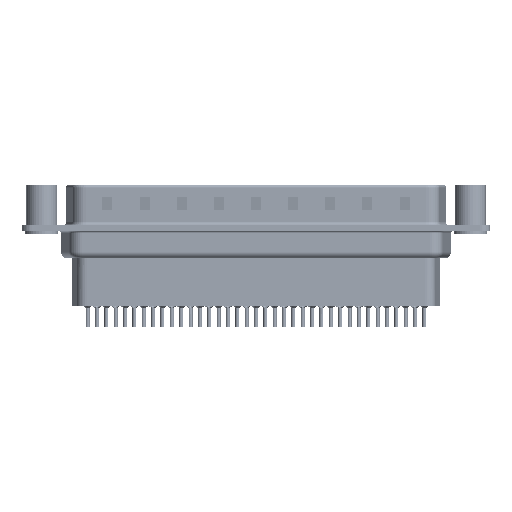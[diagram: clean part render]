
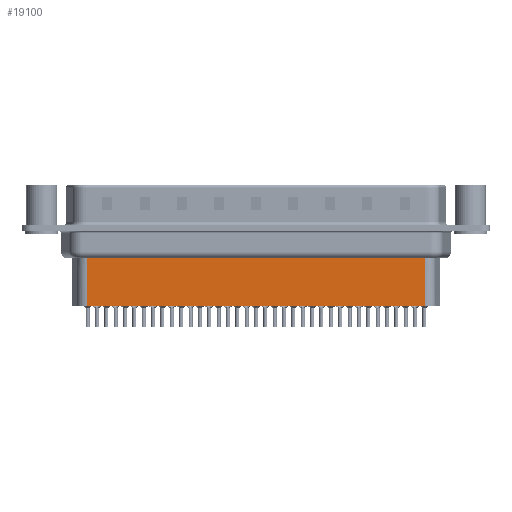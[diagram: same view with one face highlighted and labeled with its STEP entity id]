
A CAD part, front view. The second image highlights one B-rep face of the part: STEP entity #19100.
In plain terms, the highlighted planar face has unit normal (0, -1, 0).
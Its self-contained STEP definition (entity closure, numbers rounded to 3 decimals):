
#1146 = EDGE_LOOP ( 'NONE', ( #26297, #23193, #11882, #1298 ) ) ;
#1298 = ORIENTED_EDGE ( 'NONE', *, *, #6288, .F. ) ;
#3890 = VECTOR ( 'NONE', #13657, 1000. ) ;
#3902 = CARTESIAN_POINT ( 'NONE',  ( 6.706, -3.5, -3.1 ) ) ;
#4260 = CARTESIAN_POINT ( 'NONE',  ( 6.706, -3.5, -4.097 ) ) ;
#4606 = LINE ( 'NONE', #11384, #3890 ) ;
#4871 = CARTESIAN_POINT ( 'NONE',  ( 6.706, -3.5, -11.45 ) ) ;
#5815 = VERTEX_POINT ( 'NONE', #4260 ) ;
#6288 = EDGE_CURVE ( 'NONE', #29501, #21050, #11041, .T. ) ;
#6934 = CARTESIAN_POINT ( 'NONE',  ( 6.706, -3.5, -11.45 ) ) ;
#8569 = DIRECTION ( 'NONE',  ( 0., -1., 0. ) ) ;
#11041 = LINE ( 'NONE', #4871, #16388 ) ;
#11384 = CARTESIAN_POINT ( 'NONE',  ( 6.706, -3.5, -3.1 ) ) ;
#11430 = DIRECTION ( 'NONE',  ( 0., 0., -1. ) ) ;
#11882 = ORIENTED_EDGE ( 'NONE', *, *, #25477, .T. ) ;
#12043 = LINE ( 'NONE', #16840, #17436 ) ;
#12230 = DIRECTION ( 'NONE',  ( -1., 0., 0. ) ) ;
#13657 = DIRECTION ( 'NONE',  ( 0., 0., -1. ) ) ;
#13938 = LINE ( 'NONE', #25415, #26463 ) ;
#16388 = VECTOR ( 'NONE', #23358, 1000. ) ;
#16840 = CARTESIAN_POINT ( 'NONE',  ( 6.459, -3.5, -4.097 ) ) ;
#17436 = VECTOR ( 'NONE', #12230, 1000. ) ;
#19100 = ADVANCED_FACE ( 'NONE', ( #21436 ), #29514, .T. ) ;
#20316 = VERTEX_POINT ( 'NONE', #24672 ) ;
#21050 = VERTEX_POINT ( 'NONE', #6934 ) ;
#21436 = FACE_OUTER_BOUND ( 'NONE', #1146, .T. ) ;
#21588 = EDGE_CURVE ( 'NONE', #20316, #29501, #13938, .T. ) ;
#23193 = ORIENTED_EDGE ( 'NONE', *, *, #28993, .T. ) ;
#23358 = DIRECTION ( 'NONE',  ( -1., 0., 0. ) ) ;
#24672 = CARTESIAN_POINT ( 'NONE',  ( 56.794, -3.5, -4.097 ) ) ;
#24839 = DIRECTION ( 'NONE',  ( 1., 0., 0. ) ) ;
#25415 = CARTESIAN_POINT ( 'NONE',  ( 56.794, -3.5, -3.1 ) ) ;
#25477 = EDGE_CURVE ( 'NONE', #5815, #21050, #4606, .T. ) ;
#26297 = ORIENTED_EDGE ( 'NONE', *, *, #21588, .F. ) ;
#26463 = VECTOR ( 'NONE', #11430, 1000. ) ;
#27139 = AXIS2_PLACEMENT_3D ( 'NONE', #3902, #8569, #24839 ) ;
#28170 = CARTESIAN_POINT ( 'NONE',  ( 56.794, -3.5, -11.45 ) ) ;
#28993 = EDGE_CURVE ( 'NONE', #20316, #5815, #12043, .T. ) ;
#29501 = VERTEX_POINT ( 'NONE', #28170 ) ;
#29514 = PLANE ( 'NONE',  #27139 ) ;
